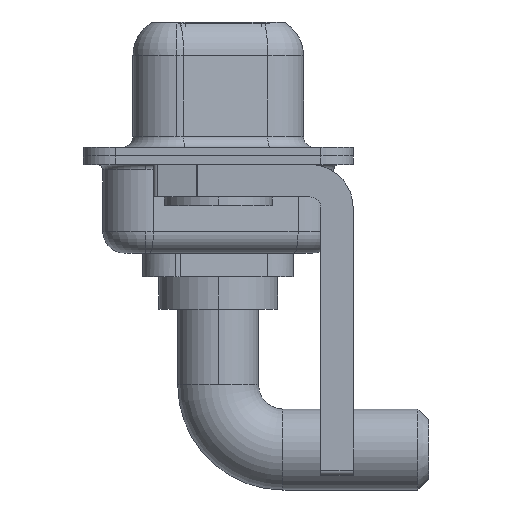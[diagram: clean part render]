
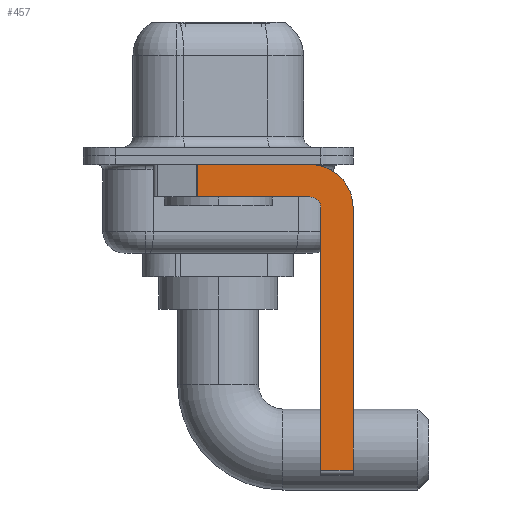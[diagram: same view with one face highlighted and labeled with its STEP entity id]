
A CAD part, left-side view. The second image highlights one B-rep face of the part: STEP entity #457.
In plain terms, the highlighted planar face has unit normal (-1, 0, 0).
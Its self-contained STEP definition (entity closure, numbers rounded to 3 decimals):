
#211 = CARTESIAN_POINT ( 'NONE',  ( -2.9, -6.25, -2.4 ) ) ;
#398 = EDGE_CURVE ( 'NONE', #951, #7034, #12493, .T. ) ;
#457 = ADVANCED_FACE ( 'NONE', ( #2204 ), #12687, .F. ) ;
#713 = CARTESIAN_POINT ( 'NONE',  ( -2.9, 0.978, -0.4 ) ) ;
#951 = VERTEX_POINT ( 'NONE', #9263 ) ;
#1157 = DIRECTION ( 'NONE',  ( 0., 0., -1. ) ) ;
#1672 = VERTEX_POINT ( 'NONE', #4880 ) ;
#1694 = CARTESIAN_POINT ( 'NONE',  ( -2.9, 3., -0.4 ) ) ;
#2194 = ORIENTED_EDGE ( 'NONE', *, *, #4147, .F. ) ;
#2204 = FACE_OUTER_BOUND ( 'NONE', #11460, .T. ) ;
#2206 = ORIENTED_EDGE ( 'NONE', *, *, #3731, .T. ) ;
#2287 = VECTOR ( 'NONE', #13217, 1000. ) ;
#2624 = CARTESIAN_POINT ( 'NONE',  ( -2.9, -4.25, -2.4 ) ) ;
#2651 = CARTESIAN_POINT ( 'NONE',  ( -2.9, -4.75, -14.8 ) ) ;
#2923 = VECTOR ( 'NONE', #7010, 1000. ) ;
#3288 = CARTESIAN_POINT ( 'NONE',  ( -2.9, -4.25, -2.4 ) ) ;
#3295 = VERTEX_POINT ( 'NONE', #3831 ) ;
#3526 = ORIENTED_EDGE ( 'NONE', *, *, #7976, .F. ) ;
#3689 = LINE ( 'NONE', #8867, #2923 ) ;
#3702 = DIRECTION ( 'NONE',  ( 0., 0., -1. ) ) ;
#3731 = EDGE_CURVE ( 'NONE', #11311, #1672, #11049, .T. ) ;
#3831 = CARTESIAN_POINT ( 'NONE',  ( -2.9, -4.75, -14.55 ) ) ;
#4147 = EDGE_CURVE ( 'NONE', #11616, #6730, #5519, .T. ) ;
#4237 = DIRECTION ( 'NONE',  ( 1., 0., 0. ) ) ;
#4301 = LINE ( 'NONE', #8192, #7260 ) ;
#4880 = CARTESIAN_POINT ( 'NONE',  ( -2.9, 0.978, -1.9 ) ) ;
#4972 = VECTOR ( 'NONE', #11396, 1000. ) ;
#5241 = EDGE_CURVE ( 'NONE', #8155, #951, #11833, .T. ) ;
#5519 = CIRCLE ( 'NONE', #12713, 0.5 ) ;
#5639 = EDGE_CURVE ( 'NONE', #6730, #1672, #3689, .T. ) ;
#5980 = ORIENTED_EDGE ( 'NONE', *, *, #5639, .F. ) ;
#6340 = CARTESIAN_POINT ( 'NONE',  ( -2.9, -4.25, -2.4 ) ) ;
#6501 = CARTESIAN_POINT ( 'NONE',  ( -2.9, -4.75, -2.4 ) ) ;
#6730 = VERTEX_POINT ( 'NONE', #12377 ) ;
#6939 = DIRECTION ( 'NONE',  ( 0., 0., -1. ) ) ;
#7010 = DIRECTION ( 'NONE',  ( 0., 1., 0. ) ) ;
#7034 = VERTEX_POINT ( 'NONE', #13048 ) ;
#7227 = EDGE_CURVE ( 'NONE', #3295, #7034, #4301, .T. ) ;
#7260 = VECTOR ( 'NONE', #9279, 1000. ) ;
#7766 = LINE ( 'NONE', #2651, #7993 ) ;
#7976 = EDGE_CURVE ( 'NONE', #11311, #8155, #12938, .T. ) ;
#7993 = VECTOR ( 'NONE', #8771, 1000. ) ;
#8155 = VERTEX_POINT ( 'NONE', #13282 ) ;
#8192 = CARTESIAN_POINT ( 'NONE',  ( -2.9, -4.25, -14.55 ) ) ;
#8771 = DIRECTION ( 'NONE',  ( 0., 0., 1. ) ) ;
#8775 = VECTOR ( 'NONE', #6939, 1000. ) ;
#8867 = CARTESIAN_POINT ( 'NONE',  ( -2.9, -4.25, -1.9 ) ) ;
#9004 = AXIS2_PLACEMENT_3D ( 'NONE', #2624, #13059, #3702 ) ;
#9036 = ORIENTED_EDGE ( 'NONE', *, *, #10723, .F. ) ;
#9052 = CARTESIAN_POINT ( 'NONE',  ( -2.9, 0.978, -1.9 ) ) ;
#9263 = CARTESIAN_POINT ( 'NONE',  ( -2.9, -6.25, -2.4 ) ) ;
#9279 = DIRECTION ( 'NONE',  ( 0., -1., 0. ) ) ;
#9343 = ORIENTED_EDGE ( 'NONE', *, *, #7227, .T. ) ;
#9552 = AXIS2_PLACEMENT_3D ( 'NONE', #6340, #4237, #1157 ) ;
#10082 = DIRECTION ( 'NONE',  ( 0., 0., 1. ) ) ;
#10723 = EDGE_CURVE ( 'NONE', #3295, #11616, #7766, .T. ) ;
#11049 = LINE ( 'NONE', #9052, #8775 ) ;
#11311 = VERTEX_POINT ( 'NONE', #713 ) ;
#11396 = DIRECTION ( 'NONE',  ( 0., 0., -1. ) ) ;
#11460 = EDGE_LOOP ( 'NONE', ( #3526, #2206, #5980, #2194, #9036, #9343, #11480, #12815 ) ) ;
#11480 = ORIENTED_EDGE ( 'NONE', *, *, #398, .F. ) ;
#11600 = DIRECTION ( 'NONE',  ( -1., 0., 0. ) ) ;
#11616 = VERTEX_POINT ( 'NONE', #6501 ) ;
#11833 = CIRCLE ( 'NONE', #9004, 2. ) ;
#12377 = CARTESIAN_POINT ( 'NONE',  ( -2.9, -4.25, -1.9 ) ) ;
#12493 = LINE ( 'NONE', #211, #4972 ) ;
#12687 = PLANE ( 'NONE',  #9552 ) ;
#12713 = AXIS2_PLACEMENT_3D ( 'NONE', #3288, #11600, #10082 ) ;
#12815 = ORIENTED_EDGE ( 'NONE', *, *, #5241, .F. ) ;
#12938 = LINE ( 'NONE', #1694, #2287 ) ;
#13048 = CARTESIAN_POINT ( 'NONE',  ( -2.9, -6.25, -14.55 ) ) ;
#13059 = DIRECTION ( 'NONE',  ( 1., 0., 0. ) ) ;
#13217 = DIRECTION ( 'NONE',  ( 0., -1., 0. ) ) ;
#13282 = CARTESIAN_POINT ( 'NONE',  ( -2.9, -4.25, -0.4 ) ) ;
